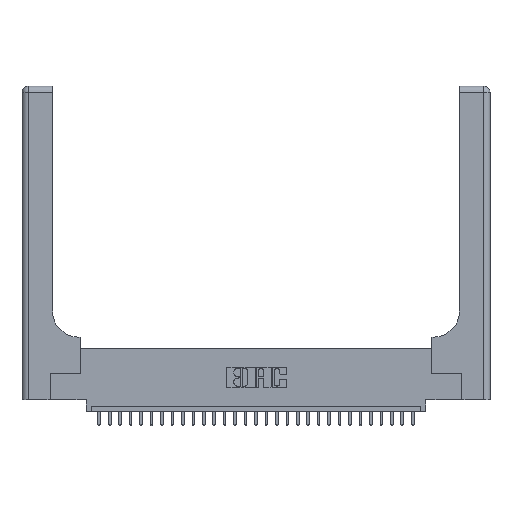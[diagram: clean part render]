
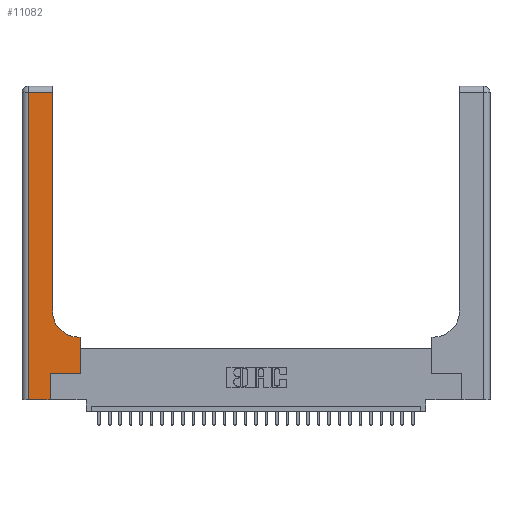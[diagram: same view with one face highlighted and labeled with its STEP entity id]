
A CAD part, top view. The second image highlights one B-rep face of the part: STEP entity #11082.
In plain terms, the highlighted planar face has unit normal (0, 0, 1).
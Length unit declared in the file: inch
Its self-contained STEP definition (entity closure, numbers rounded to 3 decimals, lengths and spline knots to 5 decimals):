
#147 = CARTESIAN_POINT ( 'NONE',  ( 0., 0., 0.37 ) ) ;
#1274 = CARTESIAN_POINT ( 'NONE',  ( 0.2915, 0.85, 0.37 ) ) ;
#1495 = EDGE_LOOP ( 'NONE', ( #9698, #8780, #20292, #29000, #23246, #4769, #14393, #27087, #4795 ) ) ;
#1700 = DIRECTION ( 'NONE',  ( -1., 0., 0. ) ) ;
#1901 = CARTESIAN_POINT ( 'NONE',  ( 0., 3., 0.37 ) ) ;
#2409 = DIRECTION ( 'NONE',  ( 1., 0., 0. ) ) ;
#3987 = DIRECTION ( 'NONE',  ( 0., 1., 0. ) ) ;
#4104 = EDGE_CURVE ( 'NONE', #18674, #30111, #18870, .T. ) ;
#4254 = DIRECTION ( 'NONE',  ( -1., 0., 0. ) ) ;
#4764 = DIRECTION ( 'NONE',  ( 0., 1., 0. ) ) ;
#4769 = ORIENTED_EDGE ( 'NONE', *, *, #14680, .T. ) ;
#4770 = LINE ( 'NONE', #147, #22592 ) ;
#4795 = ORIENTED_EDGE ( 'NONE', *, *, #4104, .T. ) ;
#4963 = CARTESIAN_POINT ( 'NONE',  ( 0.269, 0.25, 0.37 ) ) ;
#5049 = EDGE_CURVE ( 'NONE', #30111, #29292, #23973, .T. ) ;
#5135 = LINE ( 'NONE', #26746, #16743 ) ;
#5173 = EDGE_CURVE ( 'NONE', #23691, #8594, #29792, .T. ) ;
#6316 = CARTESIAN_POINT ( 'NONE',  ( 0., 2.94, 0.37 ) ) ;
#7232 = CARTESIAN_POINT ( 'NONE',  ( 0.06, 0., 0.37 ) ) ;
#7474 = CARTESIAN_POINT ( 'NONE',  ( 0.269, 0.25, 0.37 ) ) ;
#7546 = LINE ( 'NONE', #14286, #20234 ) ;
#7863 = EDGE_CURVE ( 'NONE', #18212, #18674, #19749, .T. ) ;
#8331 = VERTEX_POINT ( 'NONE', #26886 ) ;
#8579 = AXIS2_PLACEMENT_3D ( 'NONE', #17744, #11060, #22621 ) ;
#8594 = VERTEX_POINT ( 'NONE', #7474 ) ;
#8780 = ORIENTED_EDGE ( 'NONE', *, *, #28385, .T. ) ;
#9698 = ORIENTED_EDGE ( 'NONE', *, *, #5049, .T. ) ;
#10263 = CARTESIAN_POINT ( 'NONE',  ( 0.2915, 0.6, 0.37 ) ) ;
#10902 = VECTOR ( 'NONE', #3987, 39.37008 ) ;
#11060 = DIRECTION ( 'NONE',  ( 0., 0., -1. ) ) ;
#11082 = ADVANCED_FACE ( 'NONE', ( #27463 ), #20577, .F. ) ;
#12568 = CARTESIAN_POINT ( 'NONE',  ( 0.269, 0., 0.37 ) ) ;
#13110 = CARTESIAN_POINT ( 'NONE',  ( 0.5415, 0.6, 0.37 ) ) ;
#13831 = LINE ( 'NONE', #4963, #26600 ) ;
#14286 = CARTESIAN_POINT ( 'NONE',  ( 0.5585, 0.25, 0.37 ) ) ;
#14393 = ORIENTED_EDGE ( 'NONE', *, *, #16996, .T. ) ;
#14680 = EDGE_CURVE ( 'NONE', #8594, #21190, #13831, .T. ) ;
#15361 = CARTESIAN_POINT ( 'NONE',  ( 0.2915, 3., 0.37 ) ) ;
#15684 = CARTESIAN_POINT ( 'NONE',  ( 0.5585, 0.6, 0.37 ) ) ;
#16743 = VECTOR ( 'NONE', #19994, 39.37008 ) ;
#16996 = EDGE_CURVE ( 'NONE', #21190, #18212, #7546, .T. ) ;
#17744 = CARTESIAN_POINT ( 'NONE',  ( 0.5415, 0.85, 0.37 ) ) ;
#18030 = AXIS2_PLACEMENT_3D ( 'NONE', #1901, #22941, #4254 ) ;
#18212 = VERTEX_POINT ( 'NONE', #15684 ) ;
#18288 = CARTESIAN_POINT ( 'NONE',  ( 0.2915, 2.94, 0.37 ) ) ;
#18674 = VERTEX_POINT ( 'NONE', #13110 ) ;
#18748 = DIRECTION ( 'NONE',  ( 1., 0., 0. ) ) ;
#18828 = VECTOR ( 'NONE', #1700, 39.37008 ) ;
#18870 = CIRCLE ( 'NONE', #8579, 0.25 ) ;
#19749 = LINE ( 'NONE', #10263, #27430 ) ;
#19994 = DIRECTION ( 'NONE',  ( 0., -1., 0. ) ) ;
#20234 = VECTOR ( 'NONE', #4764, 39.37008 ) ;
#20292 = ORIENTED_EDGE ( 'NONE', *, *, #21448, .T. ) ;
#20577 = PLANE ( 'NONE',  #18030 ) ;
#21190 = VERTEX_POINT ( 'NONE', #23437 ) ;
#21199 = EDGE_CURVE ( 'NONE', #22010, #23691, #4770, .T. ) ;
#21448 = EDGE_CURVE ( 'NONE', #8331, #22010, #5135, .T. ) ;
#22008 = DIRECTION ( 'NONE',  ( -1., 0., 0. ) ) ;
#22010 = VERTEX_POINT ( 'NONE', #7232 ) ;
#22493 = VECTOR ( 'NONE', #22673, 39.37008 ) ;
#22592 = VECTOR ( 'NONE', #18748, 39.37008 ) ;
#22621 = DIRECTION ( 'NONE',  ( 1., 0., 0. ) ) ;
#22673 = DIRECTION ( 'NONE',  ( 0., 1., 0. ) ) ;
#22941 = DIRECTION ( 'NONE',  ( 0., 0., -1. ) ) ;
#23246 = ORIENTED_EDGE ( 'NONE', *, *, #5173, .T. ) ;
#23437 = CARTESIAN_POINT ( 'NONE',  ( 0.5585, 0.25, 0.37 ) ) ;
#23691 = VERTEX_POINT ( 'NONE', #12568 ) ;
#23973 = LINE ( 'NONE', #15361, #10902 ) ;
#25770 = LINE ( 'NONE', #6316, #18828 ) ;
#26600 = VECTOR ( 'NONE', #2409, 39.37008 ) ;
#26746 = CARTESIAN_POINT ( 'NONE',  ( 0.06, 3., 0.37 ) ) ;
#26886 = CARTESIAN_POINT ( 'NONE',  ( 0.06, 2.94, 0.37 ) ) ;
#27087 = ORIENTED_EDGE ( 'NONE', *, *, #7863, .T. ) ;
#27430 = VECTOR ( 'NONE', #22008, 39.37008 ) ;
#27463 = FACE_OUTER_BOUND ( 'NONE', #1495, .T. ) ;
#27467 = CARTESIAN_POINT ( 'NONE',  ( 0.269, 0., 0.37 ) ) ;
#28385 = EDGE_CURVE ( 'NONE', #29292, #8331, #25770, .T. ) ;
#29000 = ORIENTED_EDGE ( 'NONE', *, *, #21199, .T. ) ;
#29292 = VERTEX_POINT ( 'NONE', #18288 ) ;
#29792 = LINE ( 'NONE', #27467, #22493 ) ;
#30111 = VERTEX_POINT ( 'NONE', #1274 ) ;
